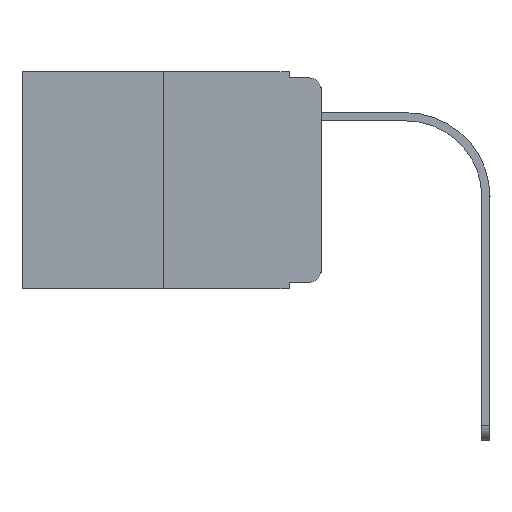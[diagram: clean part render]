
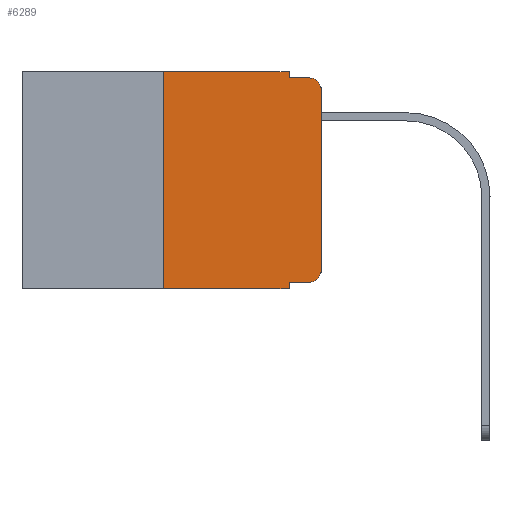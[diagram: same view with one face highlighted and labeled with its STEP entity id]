
A CAD part, left-side view. The second image highlights one B-rep face of the part: STEP entity #6289.
In plain terms, the highlighted planar face has unit normal (-1, 0, 0).
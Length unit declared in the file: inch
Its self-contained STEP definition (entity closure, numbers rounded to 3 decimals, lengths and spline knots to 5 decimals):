
#112 = DIRECTION ( 'NONE',  ( 0., -1., 0. ) ) ;
#174 = ORIENTED_EDGE ( 'NONE', *, *, #5947, .T. ) ;
#682 = CARTESIAN_POINT ( 'NONE',  ( 0., 0.473, 0. ) ) ;
#1251 = DIRECTION ( 'NONE',  ( 0., -1., 0. ) ) ;
#1656 = CARTESIAN_POINT ( 'NONE',  ( 0., 0.02, -0.333 ) ) ;
#1678 = EDGE_CURVE ( 'NONE', #8491, #9354, #5307, .T. ) ;
#1773 = VERTEX_POINT ( 'NONE', #5453 ) ;
#2225 = CARTESIAN_POINT ( 'NONE',  ( 0., 0., -0.03 ) ) ;
#2333 = CARTESIAN_POINT ( 'NONE',  ( 0., 0.25, -0.343 ) ) ;
#2344 = ORIENTED_EDGE ( 'NONE', *, *, #12444, .T. ) ;
#2374 = AXIS2_PLACEMENT_3D ( 'NONE', #3262, #6086, #8181 ) ;
#2406 = VERTEX_POINT ( 'NONE', #13750 ) ;
#2411 = CARTESIAN_POINT ( 'NONE',  ( 0., 0.051, 0. ) ) ;
#2571 = DIRECTION ( 'NONE',  ( 0., 0., -1. ) ) ;
#2608 = DIRECTION ( 'NONE',  ( 0., 0., 1. ) ) ;
#2828 = CARTESIAN_POINT ( 'NONE',  ( 0., 0.051, -0.333 ) ) ;
#3105 = ORIENTED_EDGE ( 'NONE', *, *, #10878, .F. ) ;
#3232 = CIRCLE ( 'NONE', #13051, 0.02 ) ;
#3262 = CARTESIAN_POINT ( 'NONE',  ( 0., 0.02, -0.313 ) ) ;
#3627 = AXIS2_PLACEMENT_3D ( 'NONE', #682, #4665, #12223 ) ;
#3763 = FACE_OUTER_BOUND ( 'NONE', #7201, .T. ) ;
#3790 = ORIENTED_EDGE ( 'NONE', *, *, #10914, .T. ) ;
#3913 = CARTESIAN_POINT ( 'NONE',  ( 0., 0.051, -0.343 ) ) ;
#3919 = CARTESIAN_POINT ( 'NONE',  ( 0., 0.051, 0. ) ) ;
#3954 = VERTEX_POINT ( 'NONE', #2333 ) ;
#4537 = CARTESIAN_POINT ( 'NONE',  ( 0., 0.02, -0.03 ) ) ;
#4665 = DIRECTION ( 'NONE',  ( 1., 0., 0. ) ) ;
#4737 = CARTESIAN_POINT ( 'NONE',  ( 0., 0.25, 0. ) ) ;
#4809 = CARTESIAN_POINT ( 'NONE',  ( 0., 0.051, 0. ) ) ;
#4948 = VERTEX_POINT ( 'NONE', #1656 ) ;
#5053 = VECTOR ( 'NONE', #8090, 39.37008 ) ;
#5307 = LINE ( 'NONE', #3919, #10453 ) ;
#5453 = CARTESIAN_POINT ( 'NONE',  ( 0., 0., -0.313 ) ) ;
#5781 = CARTESIAN_POINT ( 'NONE',  ( 0., 0.051, -0.01 ) ) ;
#5947 = EDGE_CURVE ( 'NONE', #3954, #9354, #9564, .T. ) ;
#6042 = EDGE_CURVE ( 'NONE', #12198, #12482, #12012, .T. ) ;
#6086 = DIRECTION ( 'NONE',  ( -1., 0., 0. ) ) ;
#6289 = ADVANCED_FACE ( 'NONE', ( #3763 ), #11102, .F. ) ;
#6690 = CARTESIAN_POINT ( 'NONE',  ( 0., 0.02, -0.01 ) ) ;
#6696 = DIRECTION ( 'NONE',  ( 0., 0., -1. ) ) ;
#6743 = CARTESIAN_POINT ( 'NONE',  ( 0., 0.051, -0.333 ) ) ;
#6832 = LINE ( 'NONE', #10894, #7035 ) ;
#6953 = VECTOR ( 'NONE', #1251, 39.37008 ) ;
#7035 = VECTOR ( 'NONE', #9918, 39.37008 ) ;
#7201 = EDGE_LOOP ( 'NONE', ( #11063, #3790, #9928, #12279, #9820, #3105, #174, #11115, #2344, #9231 ) ) ;
#7417 = VERTEX_POINT ( 'NONE', #2225 ) ;
#7470 = DIRECTION ( 'NONE',  ( 0., -1., 0. ) ) ;
#7875 = VERTEX_POINT ( 'NONE', #6690 ) ;
#7909 = EDGE_CURVE ( 'NONE', #12482, #2406, #9979, .T. ) ;
#8090 = DIRECTION ( 'NONE',  ( 0., -1., 0. ) ) ;
#8181 = DIRECTION ( 'NONE',  ( 0., 0., -1. ) ) ;
#8491 = VERTEX_POINT ( 'NONE', #2828 ) ;
#9075 = CIRCLE ( 'NONE', #2374, 0.02 ) ;
#9209 = LINE ( 'NONE', #5781, #5053 ) ;
#9231 = ORIENTED_EDGE ( 'NONE', *, *, #11835, .T. ) ;
#9354 = VERTEX_POINT ( 'NONE', #3913 ) ;
#9356 = CARTESIAN_POINT ( 'NONE',  ( 0., 0.473, -0.343 ) ) ;
#9564 = LINE ( 'NONE', #9356, #13692 ) ;
#9627 = VECTOR ( 'NONE', #2571, 39.37008 ) ;
#9685 = LINE ( 'NONE', #6743, #9745 ) ;
#9745 = VECTOR ( 'NONE', #112, 39.37008 ) ;
#9768 = CARTESIAN_POINT ( 'NONE',  ( 0., 0.473, 0. ) ) ;
#9820 = ORIENTED_EDGE ( 'NONE', *, *, #6042, .F. ) ;
#9918 = DIRECTION ( 'NONE',  ( 0., 0., 1. ) ) ;
#9928 = ORIENTED_EDGE ( 'NONE', *, *, #12181, .F. ) ;
#9979 = LINE ( 'NONE', #4809, #9627 ) ;
#10453 = VECTOR ( 'NONE', #12446, 39.37008 ) ;
#10878 = EDGE_CURVE ( 'NONE', #3954, #12198, #6832, .T. ) ;
#10894 = CARTESIAN_POINT ( 'NONE',  ( 0., 0.25, 0. ) ) ;
#10914 = EDGE_CURVE ( 'NONE', #7417, #7875, #3232, .T. ) ;
#10925 = CARTESIAN_POINT ( 'NONE',  ( 0., 0., 0. ) ) ;
#11063 = ORIENTED_EDGE ( 'NONE', *, *, #11659, .T. ) ;
#11102 = PLANE ( 'NONE',  #3627 ) ;
#11115 = ORIENTED_EDGE ( 'NONE', *, *, #1678, .F. ) ;
#11659 = EDGE_CURVE ( 'NONE', #1773, #7417, #13090, .T. ) ;
#11742 = VECTOR ( 'NONE', #2608, 39.37008 ) ;
#11835 = EDGE_CURVE ( 'NONE', #4948, #1773, #9075, .T. ) ;
#12012 = LINE ( 'NONE', #9768, #6953 ) ;
#12181 = EDGE_CURVE ( 'NONE', #2406, #7875, #9209, .T. ) ;
#12198 = VERTEX_POINT ( 'NONE', #4737 ) ;
#12223 = DIRECTION ( 'NONE',  ( 0., 0., -1. ) ) ;
#12225 = DIRECTION ( 'NONE',  ( -1., 0., 0. ) ) ;
#12279 = ORIENTED_EDGE ( 'NONE', *, *, #7909, .F. ) ;
#12444 = EDGE_CURVE ( 'NONE', #8491, #4948, #9685, .T. ) ;
#12446 = DIRECTION ( 'NONE',  ( 0., 0., -1. ) ) ;
#12482 = VERTEX_POINT ( 'NONE', #2411 ) ;
#13051 = AXIS2_PLACEMENT_3D ( 'NONE', #4537, #12225, #6696 ) ;
#13090 = LINE ( 'NONE', #10925, #11742 ) ;
#13692 = VECTOR ( 'NONE', #7470, 39.37008 ) ;
#13750 = CARTESIAN_POINT ( 'NONE',  ( 0., 0.051, -0.01 ) ) ;
